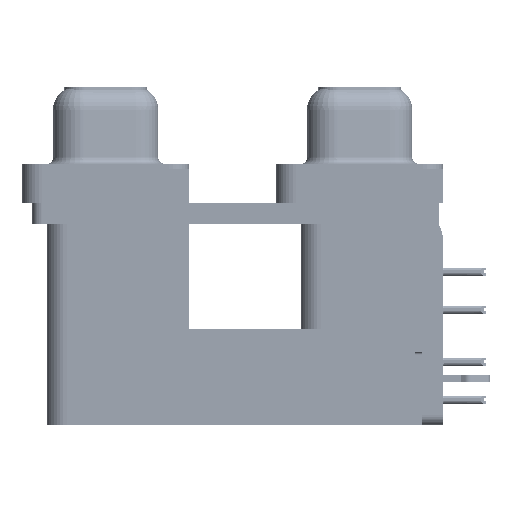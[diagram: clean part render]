
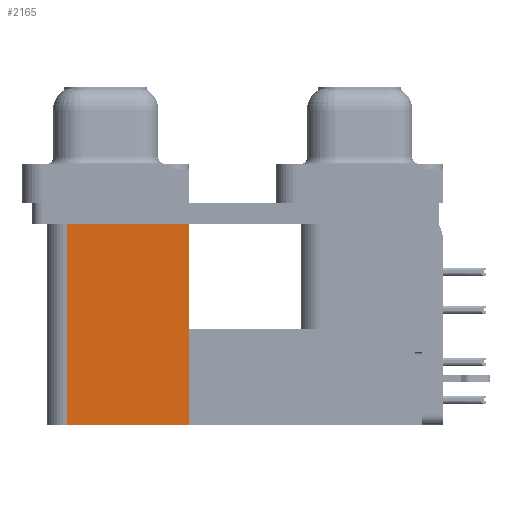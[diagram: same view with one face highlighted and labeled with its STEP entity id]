
A CAD part, left-side view. The second image highlights one B-rep face of the part: STEP entity #2165.
In plain terms, the highlighted planar face has unit normal (-1, 0, 0).
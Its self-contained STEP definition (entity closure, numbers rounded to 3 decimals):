
#2165 = ADVANCED_FACE ( 'NONE', ( #17915 ), #51048, .F. ) ;
#3066 = CARTESIAN_POINT ( 'NONE',  ( 3.7, 12.775, -19.2 ) ) ;
#3570 = LINE ( 'NONE', #55660, #31974 ) ;
#5384 = CARTESIAN_POINT ( 'NONE',  ( 3.7, 21.975, -2.5 ) ) ;
#5975 = VERTEX_POINT ( 'NONE', #29554 ) ;
#6462 = CARTESIAN_POINT ( 'NONE',  ( 3.7, 21.975, -19.2 ) ) ;
#7834 = CARTESIAN_POINT ( 'NONE',  ( 3.7, 12.775, -19.2 ) ) ;
#7993 = EDGE_LOOP ( 'NONE', ( #17145, #55136, #27699, #23482 ) ) ;
#11560 = EDGE_CURVE ( 'NONE', #46241, #44533, #3570, .T. ) ;
#12425 = DIRECTION ( 'NONE',  ( 0., 0., 1. ) ) ;
#16704 = AXIS2_PLACEMENT_3D ( 'NONE', #7834, #46313, #45682 ) ;
#17145 = ORIENTED_EDGE ( 'NONE', *, *, #11560, .T. ) ;
#17915 = FACE_OUTER_BOUND ( 'NONE', #7993, .T. ) ;
#22190 = LINE ( 'NONE', #55671, #30371 ) ;
#22647 = EDGE_CURVE ( 'NONE', #26065, #5975, #45170, .T. ) ;
#22790 = VECTOR ( 'NONE', #59493, 1000. ) ;
#23482 = ORIENTED_EDGE ( 'NONE', *, *, #50026, .T. ) ;
#24987 = CARTESIAN_POINT ( 'NONE',  ( 3.7, 12.775, -19.2 ) ) ;
#25395 = LINE ( 'NONE', #6462, #22790 ) ;
#26065 = VERTEX_POINT ( 'NONE', #3066 ) ;
#27699 = ORIENTED_EDGE ( 'NONE', *, *, #22647, .F. ) ;
#27945 = VECTOR ( 'NONE', #39504, 1000. ) ;
#29554 = CARTESIAN_POINT ( 'NONE',  ( 3.7, 21.975, -19.2 ) ) ;
#30371 = VECTOR ( 'NONE', #12425, 1000. ) ;
#31974 = VECTOR ( 'NONE', #60399, 1000. ) ;
#39504 = DIRECTION ( 'NONE',  ( 0., 1., 0. ) ) ;
#43583 = EDGE_CURVE ( 'NONE', #5975, #44533, #25395, .T. ) ;
#44533 = VERTEX_POINT ( 'NONE', #5384 ) ;
#45170 = LINE ( 'NONE', #24987, #27945 ) ;
#45682 = DIRECTION ( 'NONE',  ( 0., 1., 0. ) ) ;
#46241 = VERTEX_POINT ( 'NONE', #52023 ) ;
#46313 = DIRECTION ( 'NONE',  ( 1., 0., 0. ) ) ;
#50026 = EDGE_CURVE ( 'NONE', #26065, #46241, #22190, .T. ) ;
#51048 = PLANE ( 'NONE',  #16704 ) ;
#52023 = CARTESIAN_POINT ( 'NONE',  ( 3.7, 12.775, -2.5 ) ) ;
#55136 = ORIENTED_EDGE ( 'NONE', *, *, #43583, .F. ) ;
#55660 = CARTESIAN_POINT ( 'NONE',  ( 3.7, 12.775, -2.5 ) ) ;
#55671 = CARTESIAN_POINT ( 'NONE',  ( 3.7, 12.775, -19.2 ) ) ;
#59493 = DIRECTION ( 'NONE',  ( 0., 0., 1. ) ) ;
#60399 = DIRECTION ( 'NONE',  ( 0., 1., 0. ) ) ;
